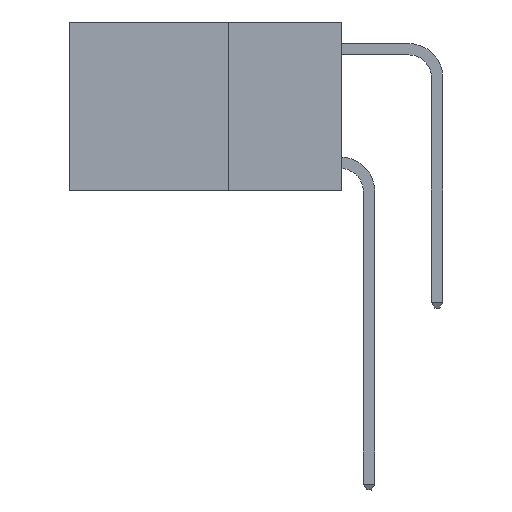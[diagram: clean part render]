
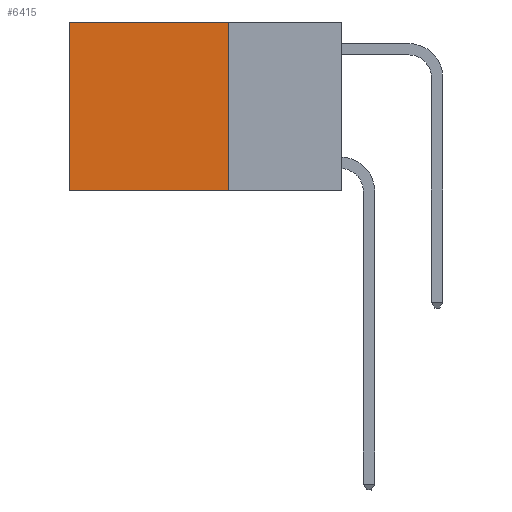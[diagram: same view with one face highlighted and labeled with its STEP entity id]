
A CAD part, left-side view. The second image highlights one B-rep face of the part: STEP entity #6415.
In plain terms, the highlighted planar face has unit normal (-1, 0, 0).
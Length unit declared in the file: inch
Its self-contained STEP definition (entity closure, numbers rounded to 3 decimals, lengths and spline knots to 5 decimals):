
#199 = ORIENTED_EDGE ( 'NONE', *, *, #10788, .T. ) ;
#653 = VECTOR ( 'NONE', #8924, 39.37008 ) ;
#1030 = LINE ( 'NONE', #2819, #653 ) ;
#1342 = LINE ( 'NONE', #8428, #13520 ) ;
#2819 = CARTESIAN_POINT ( 'NONE',  ( 0.2625, 0.6, 0. ) ) ;
#3207 = ORIENTED_EDGE ( 'NONE', *, *, #4547, .T. ) ;
#3455 = DIRECTION ( 'NONE',  ( 0., 0., -1. ) ) ;
#3922 = VECTOR ( 'NONE', #4803, 39.37008 ) ;
#4524 = AXIS2_PLACEMENT_3D ( 'NONE', #15571, #10721, #3455 ) ;
#4547 = EDGE_CURVE ( 'NONE', #15724, #14075, #1030, .T. ) ;
#4803 = DIRECTION ( 'NONE',  ( 0., 1., 0. ) ) ;
#6415 = ADVANCED_FACE ( 'NONE', ( #7692 ), #9492, .F. ) ;
#6926 = VECTOR ( 'NONE', #9955, 39.37008 ) ;
#7153 = LINE ( 'NONE', #13302, #3922 ) ;
#7336 = EDGE_CURVE ( 'NONE', #9998, #14910, #13387, .T. ) ;
#7692 = FACE_OUTER_BOUND ( 'NONE', #9721, .T. ) ;
#8305 = CARTESIAN_POINT ( 'NONE',  ( 0.2625, 0.25, 0. ) ) ;
#8428 = CARTESIAN_POINT ( 'NONE',  ( 0.2625, 0.25, 0. ) ) ;
#8924 = DIRECTION ( 'NONE',  ( 0., 0., -1. ) ) ;
#9492 = PLANE ( 'NONE',  #4524 ) ;
#9721 = EDGE_LOOP ( 'NONE', ( #3207, #10386, #12167, #199 ) ) ;
#9955 = DIRECTION ( 'NONE',  ( 0., 0., -1. ) ) ;
#9998 = VERTEX_POINT ( 'NONE', #8305 ) ;
#10386 = ORIENTED_EDGE ( 'NONE', *, *, #14160, .F. ) ;
#10721 = DIRECTION ( 'NONE',  ( 1., 0., 0. ) ) ;
#10788 = EDGE_CURVE ( 'NONE', #9998, #15724, #1342, .T. ) ;
#12167 = ORIENTED_EDGE ( 'NONE', *, *, #7336, .F. ) ;
#12674 = CARTESIAN_POINT ( 'NONE',  ( 0.2625, 0.6, 0. ) ) ;
#13302 = CARTESIAN_POINT ( 'NONE',  ( 0.2625, 0.25, -0.37 ) ) ;
#13387 = LINE ( 'NONE', #14828, #6926 ) ;
#13520 = VECTOR ( 'NONE', #15718, 39.37008 ) ;
#13680 = CARTESIAN_POINT ( 'NONE',  ( 0.2625, 0.25, -0.37 ) ) ;
#14075 = VERTEX_POINT ( 'NONE', #14350 ) ;
#14160 = EDGE_CURVE ( 'NONE', #14910, #14075, #7153, .T. ) ;
#14350 = CARTESIAN_POINT ( 'NONE',  ( 0.2625, 0.6, -0.37 ) ) ;
#14828 = CARTESIAN_POINT ( 'NONE',  ( 0.2625, 0.25, 0. ) ) ;
#14910 = VERTEX_POINT ( 'NONE', #13680 ) ;
#15571 = CARTESIAN_POINT ( 'NONE',  ( 0.2625, 0.25, 0. ) ) ;
#15718 = DIRECTION ( 'NONE',  ( 0., 1., 0. ) ) ;
#15724 = VERTEX_POINT ( 'NONE', #12674 ) ;
